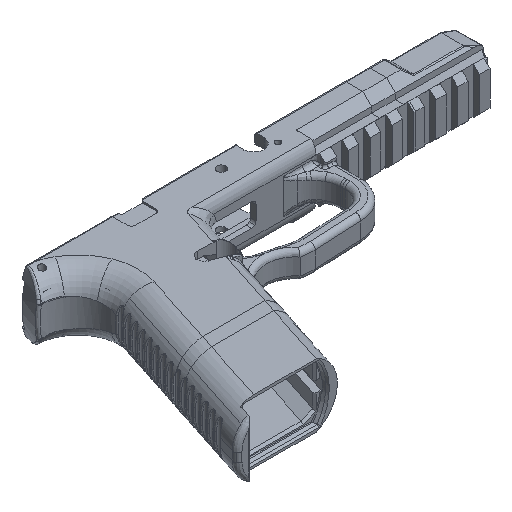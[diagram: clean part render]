
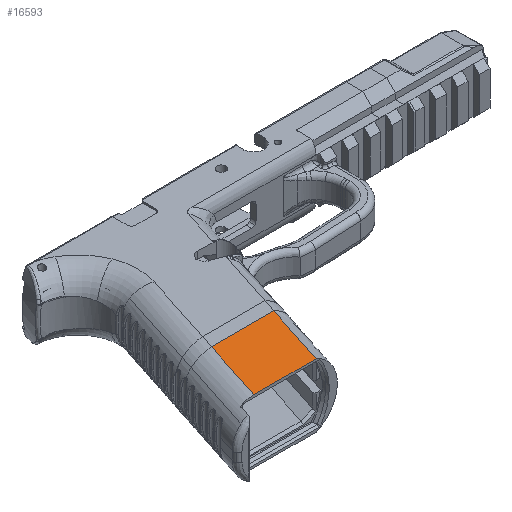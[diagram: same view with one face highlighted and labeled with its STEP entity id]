
A CAD part, isometric view. The second image highlights one B-rep face of the part: STEP entity #16593.
In plain terms, the highlighted planar face has unit normal (0, 0, 1).
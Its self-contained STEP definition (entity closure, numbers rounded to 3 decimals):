
#3321 = DIRECTION ( 'NONE',  ( 0., 0., -1. ) ) ;
#3764 = CARTESIAN_POINT ( 'NONE',  ( -98.922, 49.475, -5. ) ) ;
#3964 = VECTOR ( 'NONE', #6675, 1000. ) ;
#4199 = CARTESIAN_POINT ( 'NONE',  ( -48.777, -25.479, -5. ) ) ;
#4926 = EDGE_CURVE ( 'NONE', #27490, #27095, #40349, .T. ) ;
#5479 = VECTOR ( 'NONE', #24974, 1000. ) ;
#5596 = CARTESIAN_POINT ( 'NONE',  ( -22.913, 21.838, -5. ) ) ;
#6675 = DIRECTION ( 'NONE',  ( -1., 0., 0. ) ) ;
#6994 = CARTESIAN_POINT ( 'NONE',  ( -62.55, -12.565, -5. ) ) ;
#7273 = VERTEX_POINT ( 'NONE', #16845 ) ;
#8615 = EDGE_CURVE ( 'NONE', #27490, #37100, #11081, .T. ) ;
#10478 = ORIENTED_EDGE ( 'NONE', *, *, #25732, .F. ) ;
#11081 = LINE ( 'NONE', #4199, #32360 ) ;
#12340 = AXIS2_PLACEMENT_3D ( 'NONE', #3764, #3321, #23766 ) ;
#16592 = EDGE_CURVE ( 'NONE', #7273, #37100, #27025, .T. ) ;
#16593 = ADVANCED_FACE ( 'NONE', ( #32815 ), #40148, .F. ) ;
#16721 = ORIENTED_EDGE ( 'NONE', *, *, #16592, .F. ) ;
#16845 = CARTESIAN_POINT ( 'NONE',  ( -76.055, -54.129, -5. ) ) ;
#18124 = CARTESIAN_POINT ( 'NONE',  ( -38.287, -25.479, -5. ) ) ;
#20178 = ORIENTED_EDGE ( 'NONE', *, *, #4926, .F. ) ;
#23766 = DIRECTION ( 'NONE',  ( 0., -1., 0. ) ) ;
#24974 = DIRECTION ( 'NONE',  ( -0.309, -0.951, 0. ) ) ;
#25588 = EDGE_LOOP ( 'NONE', ( #32840, #16721, #10478, #20178 ) ) ;
#25732 = EDGE_CURVE ( 'NONE', #27095, #7273, #32939, .T. ) ;
#27025 = LINE ( 'NONE', #6994, #42629 ) ;
#27095 = VERTEX_POINT ( 'NONE', #31836 ) ;
#27490 = VERTEX_POINT ( 'NONE', #18124 ) ;
#30451 = DIRECTION ( 'NONE',  ( 0.309, 0.951, 0. ) ) ;
#31836 = CARTESIAN_POINT ( 'NONE',  ( -47.596, -54.129, -5. ) ) ;
#32360 = VECTOR ( 'NONE', #37340, 1000. ) ;
#32815 = FACE_OUTER_BOUND ( 'NONE', #25588, .T. ) ;
#32840 = ORIENTED_EDGE ( 'NONE', *, *, #8615, .T. ) ;
#32939 = LINE ( 'NONE', #39621, #3964 ) ;
#34234 = CARTESIAN_POINT ( 'NONE',  ( -66.746, -25.479, -5. ) ) ;
#37100 = VERTEX_POINT ( 'NONE', #34234 ) ;
#37340 = DIRECTION ( 'NONE',  ( -1., 0., 0. ) ) ;
#39621 = CARTESIAN_POINT ( 'NONE',  ( -67.72, -54.129, -5. ) ) ;
#40148 = PLANE ( 'NONE',  #12340 ) ;
#40349 = LINE ( 'NONE', #5596, #5479 ) ;
#42629 = VECTOR ( 'NONE', #30451, 1000. ) ;
